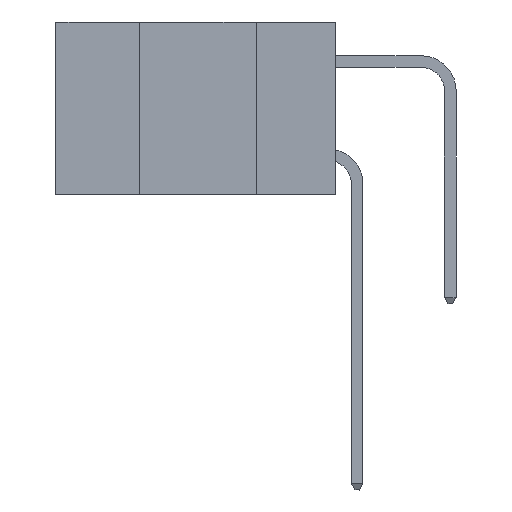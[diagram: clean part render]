
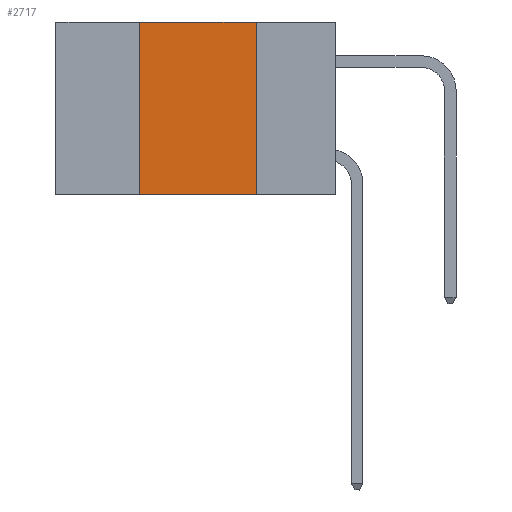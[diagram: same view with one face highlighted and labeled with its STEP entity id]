
A CAD part, left-side view. The second image highlights one B-rep face of the part: STEP entity #2717.
In plain terms, the highlighted planar face has unit normal (-1, 0, 0).
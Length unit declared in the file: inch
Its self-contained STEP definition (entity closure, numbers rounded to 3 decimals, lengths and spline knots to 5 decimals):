
#285 = VERTEX_POINT ( 'NONE', #6106 ) ;
#610 = CARTESIAN_POINT ( 'NONE',  ( 0., 0.6, 0. ) ) ;
#1234 = VECTOR ( 'NONE', #11440, 39.37008 ) ;
#2222 = DIRECTION ( 'NONE',  ( 1., 0., 0. ) ) ;
#2268 = VECTOR ( 'NONE', #5326, 39.37008 ) ;
#2666 = CARTESIAN_POINT ( 'NONE',  ( 0., 0.17, -0.37 ) ) ;
#2717 = ADVANCED_FACE ( 'NONE', ( #8748 ), #5388, .F. ) ;
#3425 = EDGE_CURVE ( 'NONE', #285, #11102, #5248, .T. ) ;
#4560 = VERTEX_POINT ( 'NONE', #7753 ) ;
#4727 = VECTOR ( 'NONE', #10250, 39.37008 ) ;
#5090 = VERTEX_POINT ( 'NONE', #13521 ) ;
#5248 = LINE ( 'NONE', #15730, #4727 ) ;
#5326 = DIRECTION ( 'NONE',  ( 0., -1., 0. ) ) ;
#5388 = PLANE ( 'NONE',  #18982 ) ;
#6106 = CARTESIAN_POINT ( 'NONE',  ( 0., 0.17, 0. ) ) ;
#7253 = ORIENTED_EDGE ( 'NONE', *, *, #3425, .F. ) ;
#7386 = ORIENTED_EDGE ( 'NONE', *, *, #16024, .F. ) ;
#7753 = CARTESIAN_POINT ( 'NONE',  ( 0., 0.42, -0.37 ) ) ;
#8476 = CARTESIAN_POINT ( 'NONE',  ( 0., 0.6, -0.37 ) ) ;
#8610 = EDGE_CURVE ( 'NONE', #4560, #11102, #15059, .T. ) ;
#8748 = FACE_OUTER_BOUND ( 'NONE', #16257, .T. ) ;
#8855 = DIRECTION ( 'NONE',  ( 0., 0., -1. ) ) ;
#9589 = VECTOR ( 'NONE', #20430, 39.37008 ) ;
#10250 = DIRECTION ( 'NONE',  ( 0., 0., -1. ) ) ;
#10615 = CARTESIAN_POINT ( 'NONE',  ( 0., 0.42, 0. ) ) ;
#11102 = VERTEX_POINT ( 'NONE', #2666 ) ;
#11440 = DIRECTION ( 'NONE',  ( 0., -1., 0. ) ) ;
#13521 = CARTESIAN_POINT ( 'NONE',  ( 0., 0.42, 0. ) ) ;
#13788 = LINE ( 'NONE', #10615, #9589 ) ;
#14447 = ORIENTED_EDGE ( 'NONE', *, *, #15411, .F. ) ;
#15059 = LINE ( 'NONE', #8476, #2268 ) ;
#15411 = EDGE_CURVE ( 'NONE', #5090, #285, #16475, .T. ) ;
#15730 = CARTESIAN_POINT ( 'NONE',  ( 0., 0.17, 0. ) ) ;
#16024 = EDGE_CURVE ( 'NONE', #4560, #5090, #13788, .T. ) ;
#16257 = EDGE_LOOP ( 'NONE', ( #7253, #14447, #7386, #17167 ) ) ;
#16475 = LINE ( 'NONE', #18093, #1234 ) ;
#17167 = ORIENTED_EDGE ( 'NONE', *, *, #8610, .T. ) ;
#18093 = CARTESIAN_POINT ( 'NONE',  ( 0., 0.6, 0. ) ) ;
#18982 = AXIS2_PLACEMENT_3D ( 'NONE', #610, #2222, #8855 ) ;
#20430 = DIRECTION ( 'NONE',  ( 0., 0., 1. ) ) ;
